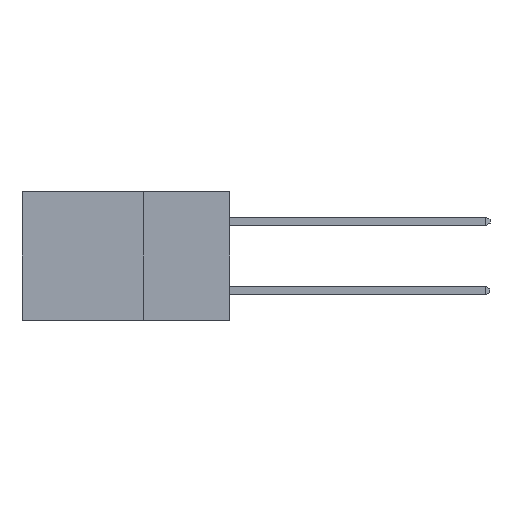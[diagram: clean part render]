
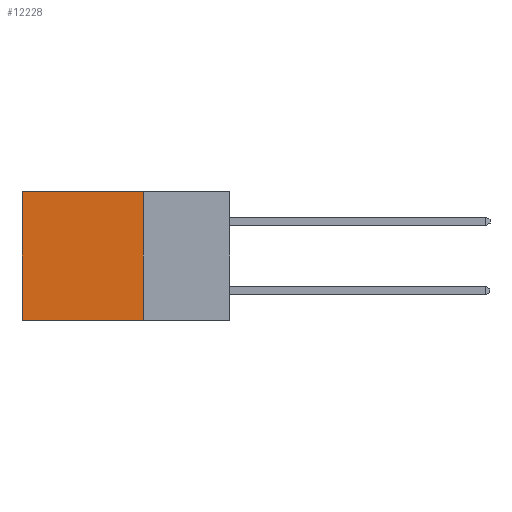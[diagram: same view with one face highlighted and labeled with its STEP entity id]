
A CAD part, left-side view. The second image highlights one B-rep face of the part: STEP entity #12228.
In plain terms, the highlighted planar face has unit normal (-1, 0, 0).
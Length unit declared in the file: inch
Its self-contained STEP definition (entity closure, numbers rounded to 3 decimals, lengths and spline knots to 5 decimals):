
#63 = AXIS2_PLACEMENT_3D ( 'NONE', #4622, #7862, #1331 ) ;
#286 = VECTOR ( 'NONE', #9752, 39.37008 ) ;
#895 = EDGE_CURVE ( 'NONE', #4589, #12539, #1967, .T. ) ;
#1068 = CARTESIAN_POINT ( 'NONE',  ( 0.298, 0.25, 0. ) ) ;
#1331 = DIRECTION ( 'NONE',  ( 0., 0., -1. ) ) ;
#1967 = LINE ( 'NONE', #12263, #12498 ) ;
#2091 = EDGE_LOOP ( 'NONE', ( #11436, #6829, #7709, #9009 ) ) ;
#2116 = DIRECTION ( 'NONE',  ( 0., 1., 0. ) ) ;
#2149 = FACE_OUTER_BOUND ( 'NONE', #2091, .T. ) ;
#3298 = LINE ( 'NONE', #12777, #6217 ) ;
#3327 = LINE ( 'NONE', #7684, #286 ) ;
#4038 = EDGE_CURVE ( 'NONE', #12539, #12317, #3298, .T. ) ;
#4589 = VERTEX_POINT ( 'NONE', #1068 ) ;
#4622 = CARTESIAN_POINT ( 'NONE',  ( 0.298, 0.25, 0. ) ) ;
#4659 = VERTEX_POINT ( 'NONE', #12504 ) ;
#5553 = DIRECTION ( 'NONE',  ( 0., 0., -1. ) ) ;
#6217 = VECTOR ( 'NONE', #12460, 39.37008 ) ;
#6829 = ORIENTED_EDGE ( 'NONE', *, *, #12081, .F. ) ;
#7613 = VECTOR ( 'NONE', #5553, 39.37008 ) ;
#7684 = CARTESIAN_POINT ( 'NONE',  ( 0.298, 0.25, -0.37 ) ) ;
#7709 = ORIENTED_EDGE ( 'NONE', *, *, #10662, .F. ) ;
#7862 = DIRECTION ( 'NONE',  ( 1., 0., 0. ) ) ;
#8369 = CARTESIAN_POINT ( 'NONE',  ( 0.298, 0.6, 0. ) ) ;
#9009 = ORIENTED_EDGE ( 'NONE', *, *, #895, .T. ) ;
#9752 = DIRECTION ( 'NONE',  ( 0., 1., 0. ) ) ;
#10662 = EDGE_CURVE ( 'NONE', #4589, #4659, #12679, .T. ) ;
#10880 = PLANE ( 'NONE',  #63 ) ;
#11052 = CARTESIAN_POINT ( 'NONE',  ( 0.298, 0.6, -0.37 ) ) ;
#11436 = ORIENTED_EDGE ( 'NONE', *, *, #4038, .T. ) ;
#11728 = CARTESIAN_POINT ( 'NONE',  ( 0.298, 0.25, 0. ) ) ;
#12081 = EDGE_CURVE ( 'NONE', #4659, #12317, #3327, .T. ) ;
#12228 = ADVANCED_FACE ( 'NONE', ( #2149 ), #10880, .F. ) ;
#12263 = CARTESIAN_POINT ( 'NONE',  ( 0.298, 0.25, 0. ) ) ;
#12317 = VERTEX_POINT ( 'NONE', #11052 ) ;
#12460 = DIRECTION ( 'NONE',  ( 0., 0., -1. ) ) ;
#12498 = VECTOR ( 'NONE', #2116, 39.37008 ) ;
#12504 = CARTESIAN_POINT ( 'NONE',  ( 0.298, 0.25, -0.37 ) ) ;
#12539 = VERTEX_POINT ( 'NONE', #8369 ) ;
#12679 = LINE ( 'NONE', #11728, #7613 ) ;
#12777 = CARTESIAN_POINT ( 'NONE',  ( 0.298, 0.6, 0. ) ) ;
